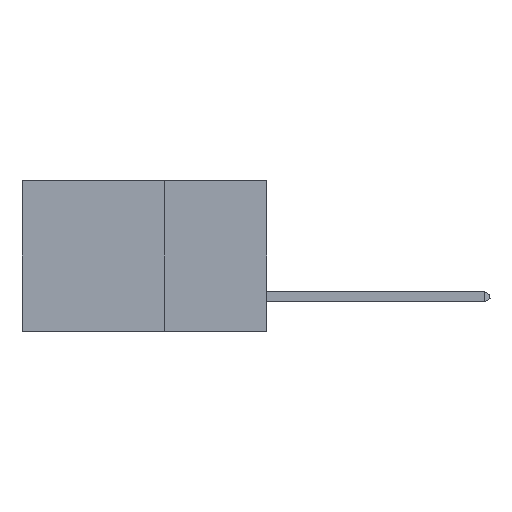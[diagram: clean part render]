
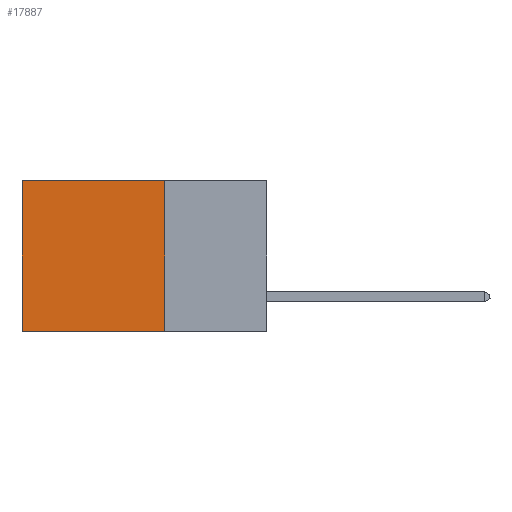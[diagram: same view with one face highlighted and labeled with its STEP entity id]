
A CAD part, left-side view. The second image highlights one B-rep face of the part: STEP entity #17887.
In plain terms, the highlighted planar face has unit normal (-1, 0, 0).
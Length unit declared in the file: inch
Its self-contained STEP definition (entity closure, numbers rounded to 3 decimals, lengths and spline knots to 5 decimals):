
#489 = VERTEX_POINT ( 'NONE', #8468 ) ;
#930 = VECTOR ( 'NONE', #2640, 39.37008 ) ;
#1315 = EDGE_LOOP ( 'NONE', ( #8544, #3078, #10341, #11864 ) ) ;
#1602 = VERTEX_POINT ( 'NONE', #12408 ) ;
#1883 = CARTESIAN_POINT ( 'NONE',  ( 0.2875, 0.25, 0. ) ) ;
#1966 = LINE ( 'NONE', #1883, #12215 ) ;
#2031 = CARTESIAN_POINT ( 'NONE',  ( 0.2875, 0.25, 0. ) ) ;
#2168 = VECTOR ( 'NONE', #2172, 39.37008 ) ;
#2172 = DIRECTION ( 'NONE',  ( 0., 0., -1. ) ) ;
#2640 = DIRECTION ( 'NONE',  ( 0., 0., -1. ) ) ;
#3078 = ORIENTED_EDGE ( 'NONE', *, *, #10682, .F. ) ;
#3283 = VERTEX_POINT ( 'NONE', #5255 ) ;
#3470 = LINE ( 'NONE', #10429, #2168 ) ;
#5059 = CARTESIAN_POINT ( 'NONE',  ( 0.2875, 0.6, 0. ) ) ;
#5255 = CARTESIAN_POINT ( 'NONE',  ( 0.2875, 0.6, -0.37 ) ) ;
#5890 = EDGE_CURVE ( 'NONE', #1602, #10106, #1966, .T. ) ;
#5912 = LINE ( 'NONE', #2031, #930 ) ;
#5987 = PLANE ( 'NONE',  #13288 ) ;
#7552 = DIRECTION ( 'NONE',  ( 0., 0., -1. ) ) ;
#7613 = DIRECTION ( 'NONE',  ( 1., 0., 0. ) ) ;
#8289 = CARTESIAN_POINT ( 'NONE',  ( 0.2875, 0.25, -0.37 ) ) ;
#8468 = CARTESIAN_POINT ( 'NONE',  ( 0.2875, 0.25, -0.37 ) ) ;
#8544 = ORIENTED_EDGE ( 'NONE', *, *, #10985, .T. ) ;
#9172 = VECTOR ( 'NONE', #14238, 39.37008 ) ;
#10106 = VERTEX_POINT ( 'NONE', #5059 ) ;
#10341 = ORIENTED_EDGE ( 'NONE', *, *, #16872, .F. ) ;
#10429 = CARTESIAN_POINT ( 'NONE',  ( 0.2875, 0.6, 0. ) ) ;
#10682 = EDGE_CURVE ( 'NONE', #489, #3283, #16350, .T. ) ;
#10985 = EDGE_CURVE ( 'NONE', #10106, #3283, #3470, .T. ) ;
#11864 = ORIENTED_EDGE ( 'NONE', *, *, #5890, .T. ) ;
#12215 = VECTOR ( 'NONE', #17375, 39.37008 ) ;
#12408 = CARTESIAN_POINT ( 'NONE',  ( 0.2875, 0.25, 0. ) ) ;
#13288 = AXIS2_PLACEMENT_3D ( 'NONE', #15893, #7613, #7552 ) ;
#13980 = FACE_OUTER_BOUND ( 'NONE', #1315, .T. ) ;
#14238 = DIRECTION ( 'NONE',  ( 0., 1., 0. ) ) ;
#15893 = CARTESIAN_POINT ( 'NONE',  ( 0.2875, 0.25, 0. ) ) ;
#16350 = LINE ( 'NONE', #8289, #9172 ) ;
#16872 = EDGE_CURVE ( 'NONE', #1602, #489, #5912, .T. ) ;
#17375 = DIRECTION ( 'NONE',  ( 0., 1., 0. ) ) ;
#17887 = ADVANCED_FACE ( 'NONE', ( #13980 ), #5987, .F. ) ;
